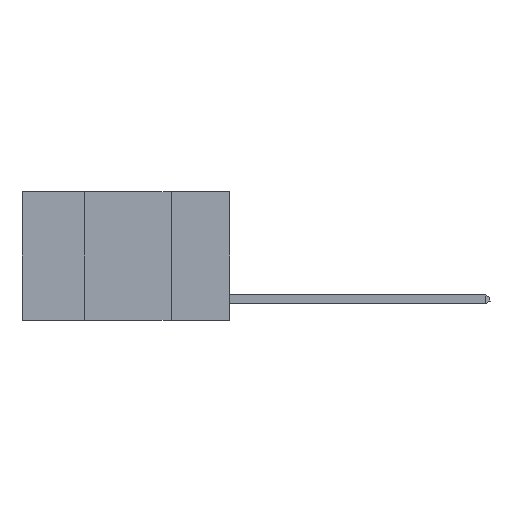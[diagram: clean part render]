
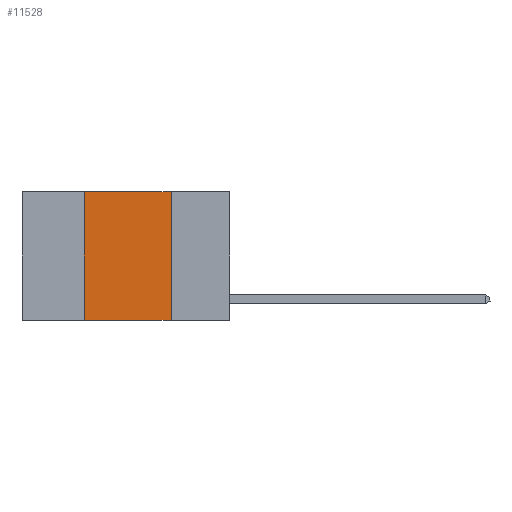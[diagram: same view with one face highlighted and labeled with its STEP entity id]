
A CAD part, left-side view. The second image highlights one B-rep face of the part: STEP entity #11528.
In plain terms, the highlighted planar face has unit normal (-1, 0, 0).
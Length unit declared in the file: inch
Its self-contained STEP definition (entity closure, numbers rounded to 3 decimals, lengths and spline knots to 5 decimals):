
#52 = CARTESIAN_POINT ( 'NONE',  ( 0., 0.17, -0.37 ) ) ;
#554 = AXIS2_PLACEMENT_3D ( 'NONE', #1969, #6265, #13672 ) ;
#742 = CARTESIAN_POINT ( 'NONE',  ( 0., 0.17, 0. ) ) ;
#1969 = CARTESIAN_POINT ( 'NONE',  ( 0., 0.6, 0. ) ) ;
#2000 = VECTOR ( 'NONE', #4402, 39.37008 ) ;
#2100 = CARTESIAN_POINT ( 'NONE',  ( 0., 0.42, -0.37 ) ) ;
#2402 = DIRECTION ( 'NONE',  ( 0., 0., -1. ) ) ;
#3158 = CARTESIAN_POINT ( 'NONE',  ( 0., 0.6, 0. ) ) ;
#3252 = EDGE_CURVE ( 'NONE', #12220, #5510, #9511, .T. ) ;
#4402 = DIRECTION ( 'NONE',  ( 0., 0., 1. ) ) ;
#4861 = LINE ( 'NONE', #12885, #2000 ) ;
#5018 = EDGE_CURVE ( 'NONE', #12243, #8054, #8059, .T. ) ;
#5510 = VERTEX_POINT ( 'NONE', #742 ) ;
#5585 = ORIENTED_EDGE ( 'NONE', *, *, #5018, .T. ) ;
#5666 = ORIENTED_EDGE ( 'NONE', *, *, #11126, .F. ) ;
#6190 = ORIENTED_EDGE ( 'NONE', *, *, #3252, .F. ) ;
#6265 = DIRECTION ( 'NONE',  ( 1., 0., 0. ) ) ;
#6295 = CARTESIAN_POINT ( 'NONE',  ( 0., 0.42, 0. ) ) ;
#6463 = ORIENTED_EDGE ( 'NONE', *, *, #7580, .F. ) ;
#6613 = LINE ( 'NONE', #7701, #9427 ) ;
#7140 = EDGE_LOOP ( 'NONE', ( #5666, #6190, #6463, #5585 ) ) ;
#7580 = EDGE_CURVE ( 'NONE', #12243, #12220, #4861, .T. ) ;
#7701 = CARTESIAN_POINT ( 'NONE',  ( 0., 0.17, 0. ) ) ;
#8054 = VERTEX_POINT ( 'NONE', #52 ) ;
#8059 = LINE ( 'NONE', #10545, #10237 ) ;
#9427 = VECTOR ( 'NONE', #2402, 39.37008 ) ;
#9511 = LINE ( 'NONE', #3158, #11333 ) ;
#10237 = VECTOR ( 'NONE', #12671, 39.37008 ) ;
#10545 = CARTESIAN_POINT ( 'NONE',  ( 0., 0.6, -0.37 ) ) ;
#11126 = EDGE_CURVE ( 'NONE', #5510, #8054, #6613, .T. ) ;
#11333 = VECTOR ( 'NONE', #13704, 39.37008 ) ;
#11528 = ADVANCED_FACE ( 'NONE', ( #12899 ), #11561, .F. ) ;
#11561 = PLANE ( 'NONE',  #554 ) ;
#12220 = VERTEX_POINT ( 'NONE', #6295 ) ;
#12243 = VERTEX_POINT ( 'NONE', #2100 ) ;
#12671 = DIRECTION ( 'NONE',  ( 0., -1., 0. ) ) ;
#12885 = CARTESIAN_POINT ( 'NONE',  ( 0., 0.42, 0. ) ) ;
#12899 = FACE_OUTER_BOUND ( 'NONE', #7140, .T. ) ;
#13672 = DIRECTION ( 'NONE',  ( 0., 0., -1. ) ) ;
#13704 = DIRECTION ( 'NONE',  ( 0., -1., 0. ) ) ;
